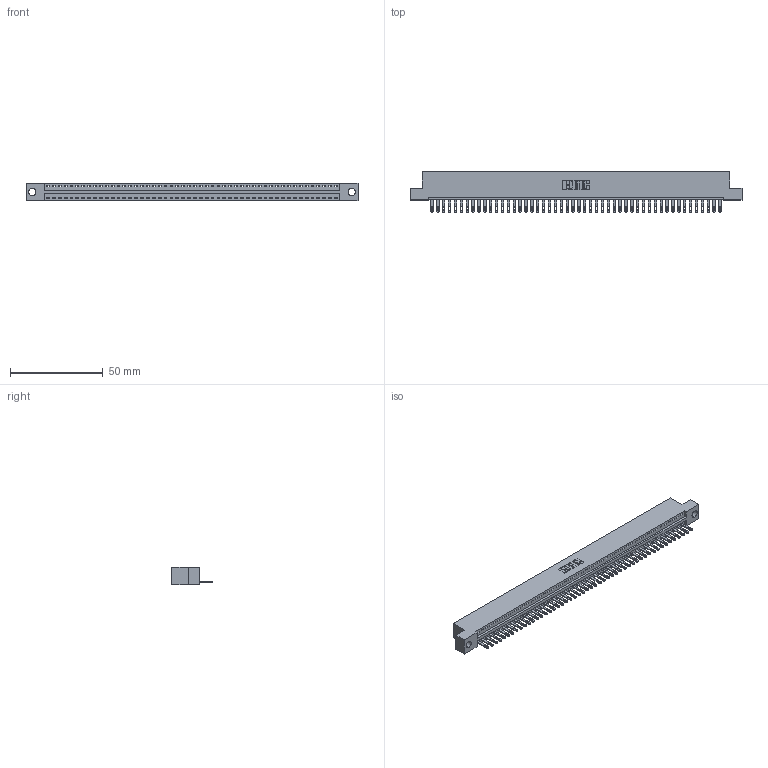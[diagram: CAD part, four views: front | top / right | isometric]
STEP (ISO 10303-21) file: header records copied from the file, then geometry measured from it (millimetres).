
FILE_DESCRIPTION (( 'STEP AP203' ), '1' );
FILE_NAME ('346-050-500-104.STEP', '2018-08-25T12:55:41', ( '' ), ( '' ), 'SwSTEP 2.0', 'SolidWorks 2016', '' );
FILE_SCHEMA (( 'CONFIG_CONTROL_DESIGN' ));
Length unit declared in the file: inch
Products named in the file (3): 346 Part_Flush Mounting Lugs - 0.156 Dia-TH; 345-292-001_345-293-100; 346-050-500-104
Assembly tree (51 placements, depth 2):
  346-050-500-104
    346 Part_Flush Mounting Lugs - 0.156 Dia-TH
    345-292-001_345-293-100  x50
Bounding box: 179.32 x 21.84 x 9.4 mm (x, y, z)
Volume: 17163.5 mm3; surface area: 21459.9 mm2
Topology: 51 solids, 51 shells, 2822 faces, 8729 edges, 5818 vertices
Faces by surface type: plane 1776, cylinder 1046
Entity records: 29887 total; most frequent: CARTESIAN_POINT 5126, ORIENTED_EDGE 5110, DIRECTION 4515, EDGE_CURVE 2555, LINE 2219, VECTOR 2219, VERTEX_POINT 1702, AXIS2_PLACEMENT_3D 1148
